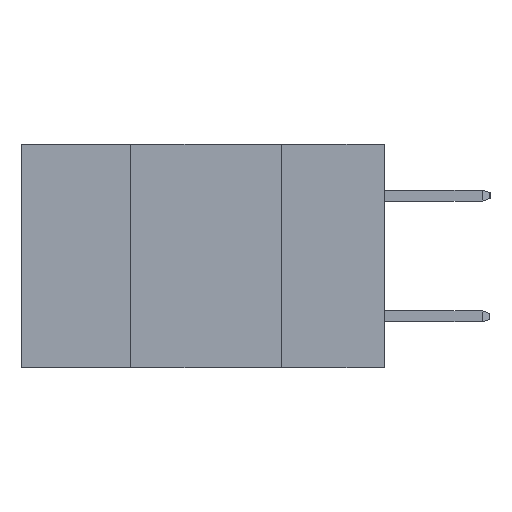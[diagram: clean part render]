
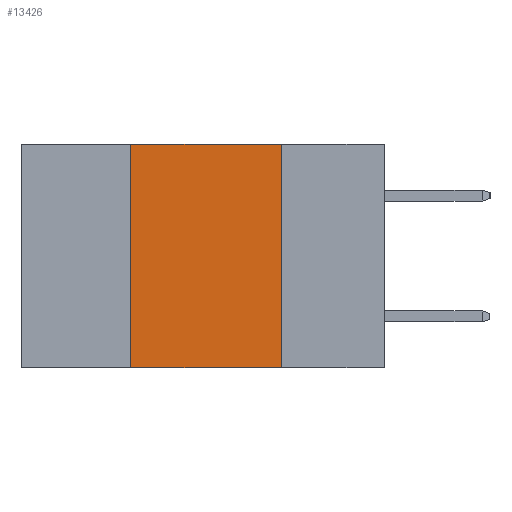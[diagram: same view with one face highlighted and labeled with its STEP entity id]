
A CAD part, left-side view. The second image highlights one B-rep face of the part: STEP entity #13426.
In plain terms, the highlighted planar face has unit normal (-1, 0, 0).
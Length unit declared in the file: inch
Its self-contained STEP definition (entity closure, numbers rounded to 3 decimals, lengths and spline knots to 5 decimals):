
#573 = CARTESIAN_POINT ( 'NONE',  ( 0., 0.17, -0.37 ) ) ;
#592 = EDGE_CURVE ( 'NONE', #10343, #8030, #11518, .T. ) ;
#605 = AXIS2_PLACEMENT_3D ( 'NONE', #744, #5336, #5120 ) ;
#744 = CARTESIAN_POINT ( 'NONE',  ( 0., 0.6, 0. ) ) ;
#1076 = CARTESIAN_POINT ( 'NONE',  ( 0., 0.17, 0. ) ) ;
#1117 = VECTOR ( 'NONE', #8170, 39.37008 ) ;
#1357 = DIRECTION ( 'NONE',  ( 0., 0., 1. ) ) ;
#1900 = FACE_OUTER_BOUND ( 'NONE', #13821, .T. ) ;
#2018 = DIRECTION ( 'NONE',  ( 0., 0., -1. ) ) ;
#2922 = LINE ( 'NONE', #15675, #12406 ) ;
#2970 = ORIENTED_EDGE ( 'NONE', *, *, #11684, .F. ) ;
#3189 = ORIENTED_EDGE ( 'NONE', *, *, #592, .F. ) ;
#3892 = VECTOR ( 'NONE', #2018, 39.37008 ) ;
#4552 = LINE ( 'NONE', #12396, #14327 ) ;
#5120 = DIRECTION ( 'NONE',  ( 0., 0., -1. ) ) ;
#5134 = CARTESIAN_POINT ( 'NONE',  ( 0., 0.6, 0. ) ) ;
#5336 = DIRECTION ( 'NONE',  ( 1., 0., 0. ) ) ;
#5744 = ORIENTED_EDGE ( 'NONE', *, *, #15739, .T. ) ;
#8030 = VERTEX_POINT ( 'NONE', #1076 ) ;
#8170 = DIRECTION ( 'NONE',  ( 0., -1., 0. ) ) ;
#8360 = VERTEX_POINT ( 'NONE', #18859 ) ;
#9701 = VERTEX_POINT ( 'NONE', #10046 ) ;
#10046 = CARTESIAN_POINT ( 'NONE',  ( 0., 0.42, -0.37 ) ) ;
#10245 = PLANE ( 'NONE',  #605 ) ;
#10343 = VERTEX_POINT ( 'NONE', #11732 ) ;
#11131 = EDGE_CURVE ( 'NONE', #9701, #10343, #2922, .T. ) ;
#11518 = LINE ( 'NONE', #5134, #1117 ) ;
#11684 = EDGE_CURVE ( 'NONE', #8030, #8360, #14876, .T. ) ;
#11732 = CARTESIAN_POINT ( 'NONE',  ( 0., 0.42, 0. ) ) ;
#12396 = CARTESIAN_POINT ( 'NONE',  ( 0., 0.6, -0.37 ) ) ;
#12406 = VECTOR ( 'NONE', #1357, 39.37008 ) ;
#13426 = ADVANCED_FACE ( 'NONE', ( #1900 ), #10245, .F. ) ;
#13750 = DIRECTION ( 'NONE',  ( 0., -1., 0. ) ) ;
#13821 = EDGE_LOOP ( 'NONE', ( #2970, #3189, #16077, #5744 ) ) ;
#14327 = VECTOR ( 'NONE', #13750, 39.37008 ) ;
#14876 = LINE ( 'NONE', #573, #3892 ) ;
#15675 = CARTESIAN_POINT ( 'NONE',  ( 0., 0.42, -0.37 ) ) ;
#15739 = EDGE_CURVE ( 'NONE', #9701, #8360, #4552, .T. ) ;
#16077 = ORIENTED_EDGE ( 'NONE', *, *, #11131, .F. ) ;
#18859 = CARTESIAN_POINT ( 'NONE',  ( 0., 0.17, -0.37 ) ) ;
